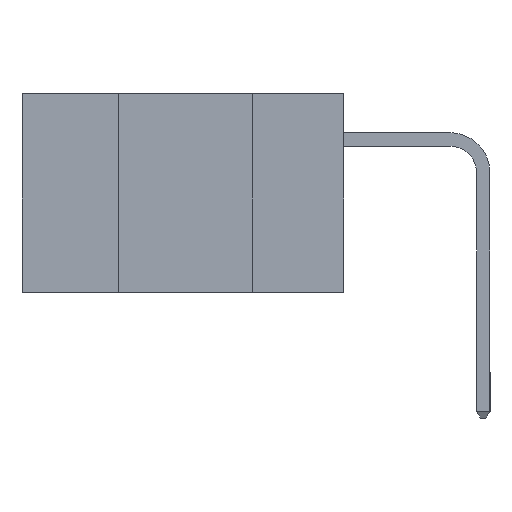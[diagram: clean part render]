
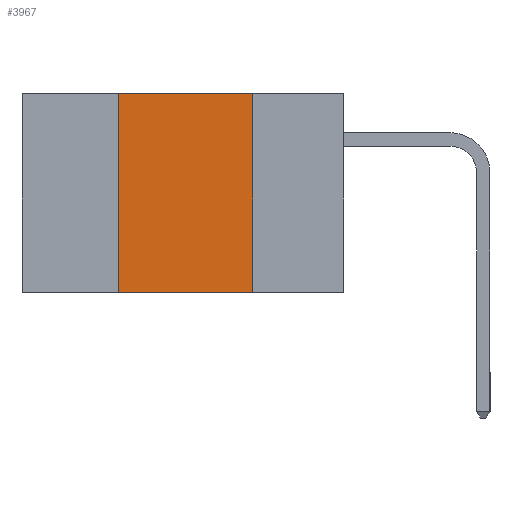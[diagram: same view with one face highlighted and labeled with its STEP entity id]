
A CAD part, left-side view. The second image highlights one B-rep face of the part: STEP entity #3967.
In plain terms, the highlighted planar face has unit normal (-1, 0, 0).
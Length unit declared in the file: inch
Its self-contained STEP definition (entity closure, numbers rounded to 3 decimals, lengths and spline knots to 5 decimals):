
#93 = DIRECTION ( 'NONE',  ( 0., -1., 0. ) ) ;
#2230 = CARTESIAN_POINT ( 'NONE',  ( 0., 0.6, 0. ) ) ;
#2547 = AXIS2_PLACEMENT_3D ( 'NONE', #13415, #14528, #14524 ) ;
#2572 = VECTOR ( 'NONE', #13029, 39.37008 ) ;
#2968 = CARTESIAN_POINT ( 'NONE',  ( 0., 0.17, -0.37 ) ) ;
#2980 = LINE ( 'NONE', #2230, #2572 ) ;
#3431 = EDGE_CURVE ( 'NONE', #10151, #14643, #7414, .T. ) ;
#3741 = DIRECTION ( 'NONE',  ( 0., 0., 1. ) ) ;
#3776 = VECTOR ( 'NONE', #93, 39.37008 ) ;
#3784 = EDGE_CURVE ( 'NONE', #14643, #8792, #2980, .T. ) ;
#3967 = ADVANCED_FACE ( 'NONE', ( #13173 ), #9114, .F. ) ;
#4025 = VECTOR ( 'NONE', #3741, 39.37008 ) ;
#4173 = ORIENTED_EDGE ( 'NONE', *, *, #11368, .F. ) ;
#5717 = ORIENTED_EDGE ( 'NONE', *, *, #3784, .F. ) ;
#5793 = CARTESIAN_POINT ( 'NONE',  ( 0., 0.42, -0.37 ) ) ;
#6474 = CARTESIAN_POINT ( 'NONE',  ( 0., 0.6, -0.37 ) ) ;
#7414 = LINE ( 'NONE', #8146, #4025 ) ;
#7464 = LINE ( 'NONE', #8678, #13231 ) ;
#7547 = ORIENTED_EDGE ( 'NONE', *, *, #3431, .F. ) ;
#7574 = VERTEX_POINT ( 'NONE', #2968 ) ;
#8146 = CARTESIAN_POINT ( 'NONE',  ( 0., 0.42, 0. ) ) ;
#8678 = CARTESIAN_POINT ( 'NONE',  ( 0., 0.17, 0. ) ) ;
#8792 = VERTEX_POINT ( 'NONE', #10700 ) ;
#9114 = PLANE ( 'NONE',  #2547 ) ;
#10151 = VERTEX_POINT ( 'NONE', #5793 ) ;
#10700 = CARTESIAN_POINT ( 'NONE',  ( 0., 0.17, 0. ) ) ;
#11278 = LINE ( 'NONE', #6474, #3776 ) ;
#11368 = EDGE_CURVE ( 'NONE', #8792, #7574, #7464, .T. ) ;
#11862 = EDGE_LOOP ( 'NONE', ( #4173, #5717, #7547, #15799 ) ) ;
#13029 = DIRECTION ( 'NONE',  ( 0., -1., 0. ) ) ;
#13173 = FACE_OUTER_BOUND ( 'NONE', #11862, .T. ) ;
#13231 = VECTOR ( 'NONE', #13512, 39.37008 ) ;
#13415 = CARTESIAN_POINT ( 'NONE',  ( 0., 0.6, 0. ) ) ;
#13479 = EDGE_CURVE ( 'NONE', #10151, #7574, #11278, .T. ) ;
#13512 = DIRECTION ( 'NONE',  ( 0., 0., -1. ) ) ;
#14524 = DIRECTION ( 'NONE',  ( 0., 0., -1. ) ) ;
#14528 = DIRECTION ( 'NONE',  ( 1., 0., 0. ) ) ;
#14643 = VERTEX_POINT ( 'NONE', #16016 ) ;
#15799 = ORIENTED_EDGE ( 'NONE', *, *, #13479, .T. ) ;
#16016 = CARTESIAN_POINT ( 'NONE',  ( 0., 0.42, 0. ) ) ;
